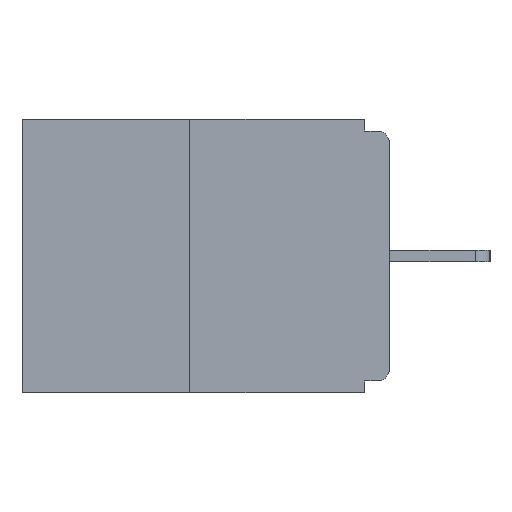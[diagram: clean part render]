
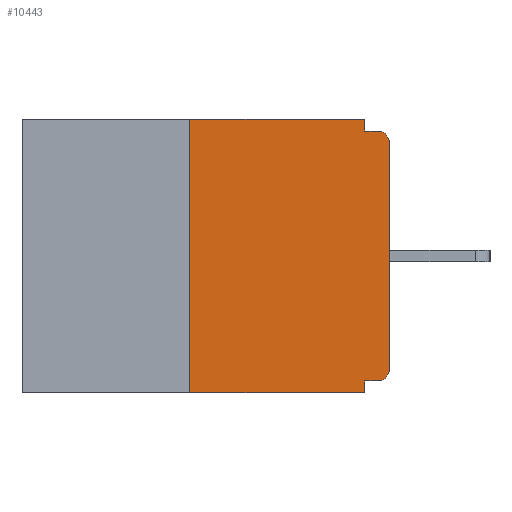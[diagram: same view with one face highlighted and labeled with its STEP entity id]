
A CAD part, left-side view. The second image highlights one B-rep face of the part: STEP entity #10443.
In plain terms, the highlighted planar face has unit normal (-1, 0, 0).
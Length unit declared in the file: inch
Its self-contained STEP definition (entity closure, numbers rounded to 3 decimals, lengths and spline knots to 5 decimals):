
#181 = VERTEX_POINT ( 'NONE', #3607 ) ;
#494 = DIRECTION ( 'NONE',  ( 0., 0., -1. ) ) ;
#500 = VERTEX_POINT ( 'NONE', #7735 ) ;
#677 = CARTESIAN_POINT ( 'NONE',  ( 0., 0., -0.313 ) ) ;
#1155 = CARTESIAN_POINT ( 'NONE',  ( 0., 0.25, -0.343 ) ) ;
#1229 = VECTOR ( 'NONE', #494, 39.37008 ) ;
#1274 = ORIENTED_EDGE ( 'NONE', *, *, #7119, .F. ) ;
#1558 = DIRECTION ( 'NONE',  ( 0., 0., 1. ) ) ;
#1709 = CARTESIAN_POINT ( 'NONE',  ( 0., 0.015, -0.03 ) ) ;
#1744 = CARTESIAN_POINT ( 'NONE',  ( 0., 0., -0.03 ) ) ;
#1879 = CARTESIAN_POINT ( 'NONE',  ( 0., 0.031, -0.328 ) ) ;
#2001 = DIRECTION ( 'NONE',  ( 0., -1., 0. ) ) ;
#2157 = CARTESIAN_POINT ( 'NONE',  ( 0., 0.031, 0. ) ) ;
#2332 = ORIENTED_EDGE ( 'NONE', *, *, #4310, .F. ) ;
#2333 = ORIENTED_EDGE ( 'NONE', *, *, #8061, .F. ) ;
#2437 = CARTESIAN_POINT ( 'NONE',  ( 0., 0.031, 0. ) ) ;
#2458 = DIRECTION ( 'NONE',  ( 0., 0., -1. ) ) ;
#2697 = FACE_OUTER_BOUND ( 'NONE', #6943, .T. ) ;
#2699 = CARTESIAN_POINT ( 'NONE',  ( 0., 0.031, -0.343 ) ) ;
#2711 = LINE ( 'NONE', #13370, #4383 ) ;
#2739 = EDGE_CURVE ( 'NONE', #8418, #8132, #4043, .T. ) ;
#3271 = CIRCLE ( 'NONE', #13540, 0.015 ) ;
#3347 = EDGE_CURVE ( 'NONE', #7296, #500, #13287, .T. ) ;
#3607 = CARTESIAN_POINT ( 'NONE',  ( 0., 0.031, -0.015 ) ) ;
#3683 = CARTESIAN_POINT ( 'NONE',  ( 0., 0.46, 0. ) ) ;
#3871 = DIRECTION ( 'NONE',  ( -1., 0., 0. ) ) ;
#3992 = ORIENTED_EDGE ( 'NONE', *, *, #7605, .F. ) ;
#4043 = LINE ( 'NONE', #9571, #7267 ) ;
#4054 = VECTOR ( 'NONE', #8995, 39.37008 ) ;
#4221 = VERTEX_POINT ( 'NONE', #677 ) ;
#4243 = DIRECTION ( 'NONE',  ( -1., 0., 0. ) ) ;
#4310 = EDGE_CURVE ( 'NONE', #181, #500, #8993, .T. ) ;
#4383 = VECTOR ( 'NONE', #1558, 39.37008 ) ;
#4525 = CARTESIAN_POINT ( 'NONE',  ( 0., 0.031, -0.343 ) ) ;
#4770 = CARTESIAN_POINT ( 'NONE',  ( 0., 0.46, 0. ) ) ;
#5442 = EDGE_CURVE ( 'NONE', #4221, #7296, #2711, .T. ) ;
#5449 = AXIS2_PLACEMENT_3D ( 'NONE', #4770, #13358, #12192 ) ;
#5678 = CARTESIAN_POINT ( 'NONE',  ( 0., 0., -0.328 ) ) ;
#5834 = LINE ( 'NONE', #2437, #10952 ) ;
#5860 = DIRECTION ( 'NONE',  ( 0., 0., 1. ) ) ;
#6487 = EDGE_CURVE ( 'NONE', #10303, #4221, #3271, .T. ) ;
#6656 = ORIENTED_EDGE ( 'NONE', *, *, #6487, .T. ) ;
#6943 = EDGE_LOOP ( 'NONE', ( #8765, #2333, #12257, #9947, #3992, #6656, #7747, #10280, #2332, #1274 ) ) ;
#7119 = EDGE_CURVE ( 'NONE', #11881, #181, #5834, .T. ) ;
#7201 = VERTEX_POINT ( 'NONE', #1879 ) ;
#7267 = VECTOR ( 'NONE', #2001, 39.37008 ) ;
#7279 = AXIS2_PLACEMENT_3D ( 'NONE', #1709, #3871, #2458 ) ;
#7296 = VERTEX_POINT ( 'NONE', #1744 ) ;
#7483 = DIRECTION ( 'NONE',  ( 0., 0., -1. ) ) ;
#7605 = EDGE_CURVE ( 'NONE', #10303, #7201, #11026, .T. ) ;
#7735 = CARTESIAN_POINT ( 'NONE',  ( 0., 0.015, -0.015 ) ) ;
#7747 = ORIENTED_EDGE ( 'NONE', *, *, #5442, .T. ) ;
#8061 = EDGE_CURVE ( 'NONE', #8418, #8283, #8908, .T. ) ;
#8132 = VERTEX_POINT ( 'NONE', #4525 ) ;
#8225 = CARTESIAN_POINT ( 'NONE',  ( 0., 0.015, -0.313 ) ) ;
#8283 = VERTEX_POINT ( 'NONE', #12761 ) ;
#8418 = VERTEX_POINT ( 'NONE', #1155 ) ;
#8765 = ORIENTED_EDGE ( 'NONE', *, *, #13571, .F. ) ;
#8908 = LINE ( 'NONE', #9821, #12778 ) ;
#8993 = LINE ( 'NONE', #10240, #9956 ) ;
#8995 = DIRECTION ( 'NONE',  ( 0., 1., 0. ) ) ;
#9571 = CARTESIAN_POINT ( 'NONE',  ( 0., 0.46, -0.343 ) ) ;
#9821 = CARTESIAN_POINT ( 'NONE',  ( 0., 0.25, 0. ) ) ;
#9947 = ORIENTED_EDGE ( 'NONE', *, *, #11556, .F. ) ;
#9956 = VECTOR ( 'NONE', #13274, 39.37008 ) ;
#9973 = LINE ( 'NONE', #3683, #11205 ) ;
#10240 = CARTESIAN_POINT ( 'NONE',  ( 0., 0., -0.015 ) ) ;
#10280 = ORIENTED_EDGE ( 'NONE', *, *, #3347, .T. ) ;
#10303 = VERTEX_POINT ( 'NONE', #12815 ) ;
#10443 = ADVANCED_FACE ( 'NONE', ( #2697 ), #12044, .F. ) ;
#10952 = VECTOR ( 'NONE', #12306, 39.37008 ) ;
#11026 = LINE ( 'NONE', #5678, #4054 ) ;
#11205 = VECTOR ( 'NONE', #12282, 39.37008 ) ;
#11556 = EDGE_CURVE ( 'NONE', #7201, #8132, #12113, .T. ) ;
#11881 = VERTEX_POINT ( 'NONE', #2157 ) ;
#12044 = PLANE ( 'NONE',  #5449 ) ;
#12113 = LINE ( 'NONE', #2699, #1229 ) ;
#12192 = DIRECTION ( 'NONE',  ( 0., 0., -1. ) ) ;
#12257 = ORIENTED_EDGE ( 'NONE', *, *, #2739, .T. ) ;
#12282 = DIRECTION ( 'NONE',  ( 0., -1., 0. ) ) ;
#12306 = DIRECTION ( 'NONE',  ( 0., 0., -1. ) ) ;
#12761 = CARTESIAN_POINT ( 'NONE',  ( 0., 0.25, 0. ) ) ;
#12778 = VECTOR ( 'NONE', #5860, 39.37008 ) ;
#12815 = CARTESIAN_POINT ( 'NONE',  ( 0., 0.015, -0.328 ) ) ;
#13274 = DIRECTION ( 'NONE',  ( 0., -1., 0. ) ) ;
#13287 = CIRCLE ( 'NONE', #7279, 0.015 ) ;
#13358 = DIRECTION ( 'NONE',  ( 1., 0., 0. ) ) ;
#13370 = CARTESIAN_POINT ( 'NONE',  ( 0., 0., 0. ) ) ;
#13540 = AXIS2_PLACEMENT_3D ( 'NONE', #8225, #4243, #7483 ) ;
#13571 = EDGE_CURVE ( 'NONE', #8283, #11881, #9973, .T. ) ;
